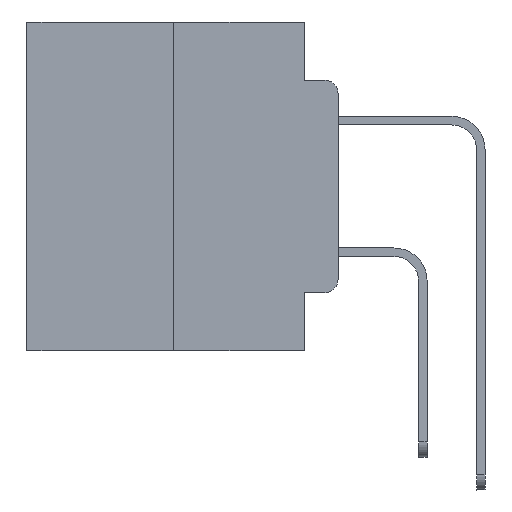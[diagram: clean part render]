
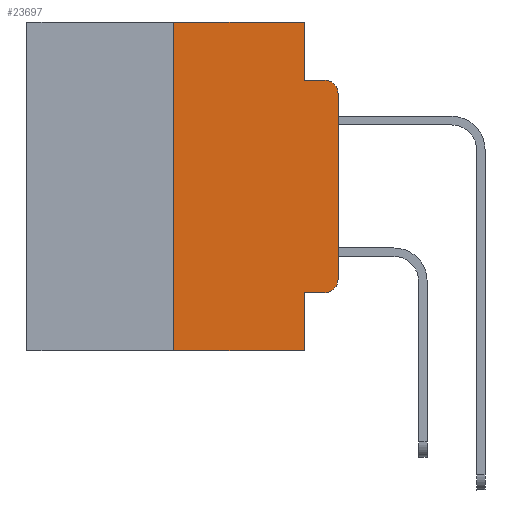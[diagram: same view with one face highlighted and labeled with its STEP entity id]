
A CAD part, left-side view. The second image highlights one B-rep face of the part: STEP entity #23697.
In plain terms, the highlighted planar face has unit normal (-1, 0, 0).
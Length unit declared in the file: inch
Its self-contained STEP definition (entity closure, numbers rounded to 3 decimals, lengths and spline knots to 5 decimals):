
#39 = CARTESIAN_POINT ( 'NONE',  ( 0., 0., -0.1085 ) ) ;
#104 = DIRECTION ( 'NONE',  ( 0., 0., -1. ) ) ;
#364 = VERTEX_POINT ( 'NONE', #5366 ) ;
#497 = CARTESIAN_POINT ( 'NONE',  ( 0., 0.473, -0.5 ) ) ;
#549 = VERTEX_POINT ( 'NONE', #11888 ) ;
#791 = DIRECTION ( 'NONE',  ( 0., 0., 1. ) ) ;
#1416 = CARTESIAN_POINT ( 'NONE',  ( 0., 0.02, -0.1085 ) ) ;
#1719 = VECTOR ( 'NONE', #791, 39.37008 ) ;
#1750 = EDGE_CURVE ( 'NONE', #549, #17195, #18834, .T. ) ;
#2584 = VECTOR ( 'NONE', #20790, 39.37008 ) ;
#2602 = LINE ( 'NONE', #497, #24653 ) ;
#3298 = ORIENTED_EDGE ( 'NONE', *, *, #20959, .F. ) ;
#3599 = DIRECTION ( 'NONE',  ( 0., 0., -1. ) ) ;
#3715 = CARTESIAN_POINT ( 'NONE',  ( 0., 0., -0.3915 ) ) ;
#3893 = CARTESIAN_POINT ( 'NONE',  ( 0., 0.051, -0.4115 ) ) ;
#4524 = VERTEX_POINT ( 'NONE', #39 ) ;
#4659 = EDGE_CURVE ( 'NONE', #364, #6423, #24624, .T. ) ;
#4721 = DIRECTION ( 'NONE',  ( 1., 0., 0. ) ) ;
#5366 = CARTESIAN_POINT ( 'NONE',  ( 0., 0.051, 0. ) ) ;
#5656 = ORIENTED_EDGE ( 'NONE', *, *, #24674, .T. ) ;
#5725 = LINE ( 'NONE', #25254, #16434 ) ;
#6086 = DIRECTION ( 'NONE',  ( 0., -1., 0. ) ) ;
#6367 = VERTEX_POINT ( 'NONE', #10604 ) ;
#6423 = VERTEX_POINT ( 'NONE', #6450 ) ;
#6450 = CARTESIAN_POINT ( 'NONE',  ( 0., 0.051, -0.0885 ) ) ;
#6804 = DIRECTION ( 'NONE',  ( 0., -1., 0. ) ) ;
#7242 = EDGE_CURVE ( 'NONE', #549, #13559, #2602, .T. ) ;
#7715 = ORIENTED_EDGE ( 'NONE', *, *, #1750, .F. ) ;
#8361 = EDGE_CURVE ( 'NONE', #17195, #364, #19679, .T. ) ;
#8904 = CARTESIAN_POINT ( 'NONE',  ( 0., 0.051, -0.0885 ) ) ;
#9070 = VERTEX_POINT ( 'NONE', #3715 ) ;
#9208 = VERTEX_POINT ( 'NONE', #27533 ) ;
#9898 = LINE ( 'NONE', #3893, #14875 ) ;
#10419 = ORIENTED_EDGE ( 'NONE', *, *, #13565, .T. ) ;
#10469 = EDGE_CURVE ( 'NONE', #6423, #10870, #12229, .T. ) ;
#10604 = CARTESIAN_POINT ( 'NONE',  ( 0., 0.051, -0.4115 ) ) ;
#10618 = CARTESIAN_POINT ( 'NONE',  ( 0., 0.02, -0.0885 ) ) ;
#10797 = EDGE_CURVE ( 'NONE', #6367, #9208, #9898, .T. ) ;
#10870 = VERTEX_POINT ( 'NONE', #10618 ) ;
#11125 = EDGE_LOOP ( 'NONE', ( #5656, #11391, #12055, #17701, #24044, #7715, #25335, #3298, #21060, #10419 ) ) ;
#11391 = ORIENTED_EDGE ( 'NONE', *, *, #20426, .T. ) ;
#11888 = CARTESIAN_POINT ( 'NONE',  ( 0., 0.25, -0.5 ) ) ;
#12055 = ORIENTED_EDGE ( 'NONE', *, *, #10469, .F. ) ;
#12229 = LINE ( 'NONE', #8904, #22877 ) ;
#12625 = VECTOR ( 'NONE', #13993, 39.37008 ) ;
#13042 = DIRECTION ( 'NONE',  ( -1., 0., 0. ) ) ;
#13264 = PLANE ( 'NONE',  #20012 ) ;
#13336 = VECTOR ( 'NONE', #17343, 39.37008 ) ;
#13559 = VERTEX_POINT ( 'NONE', #15093 ) ;
#13565 = EDGE_CURVE ( 'NONE', #9208, #9070, #22328, .T. ) ;
#13970 = CIRCLE ( 'NONE', #19260, 0.02 ) ;
#13993 = DIRECTION ( 'NONE',  ( 0., 0., -1. ) ) ;
#14875 = VECTOR ( 'NONE', #6086, 39.37008 ) ;
#15093 = CARTESIAN_POINT ( 'NONE',  ( 0., 0.051, -0.5 ) ) ;
#16434 = VECTOR ( 'NONE', #27340, 39.37008 ) ;
#16440 = DIRECTION ( 'NONE',  ( -1., 0., 0. ) ) ;
#17195 = VERTEX_POINT ( 'NONE', #22677 ) ;
#17343 = DIRECTION ( 'NONE',  ( 0., 0., -1. ) ) ;
#17437 = CARTESIAN_POINT ( 'NONE',  ( 0., 0.051, 0. ) ) ;
#17701 = ORIENTED_EDGE ( 'NONE', *, *, #4659, .F. ) ;
#18262 = LINE ( 'NONE', #26682, #12625 ) ;
#18643 = CARTESIAN_POINT ( 'NONE',  ( 0., 0.473, 0. ) ) ;
#18834 = LINE ( 'NONE', #22906, #1719 ) ;
#19188 = FACE_OUTER_BOUND ( 'NONE', #11125, .T. ) ;
#19260 = AXIS2_PLACEMENT_3D ( 'NONE', #1416, #16440, #3599 ) ;
#19679 = LINE ( 'NONE', #18643, #2584 ) ;
#19684 = DIRECTION ( 'NONE',  ( 0., 0., -1. ) ) ;
#19835 = DIRECTION ( 'NONE',  ( 0., -1., 0. ) ) ;
#20012 = AXIS2_PLACEMENT_3D ( 'NONE', #23872, #4721, #19684 ) ;
#20022 = AXIS2_PLACEMENT_3D ( 'NONE', #25741, #13042, #104 ) ;
#20426 = EDGE_CURVE ( 'NONE', #4524, #10870, #13970, .T. ) ;
#20790 = DIRECTION ( 'NONE',  ( 0., -1., 0. ) ) ;
#20959 = EDGE_CURVE ( 'NONE', #6367, #13559, #18262, .T. ) ;
#21060 = ORIENTED_EDGE ( 'NONE', *, *, #10797, .T. ) ;
#22328 = CIRCLE ( 'NONE', #20022, 0.02 ) ;
#22677 = CARTESIAN_POINT ( 'NONE',  ( 0., 0.25, 0. ) ) ;
#22877 = VECTOR ( 'NONE', #6804, 39.37008 ) ;
#22906 = CARTESIAN_POINT ( 'NONE',  ( 0., 0.25, 0. ) ) ;
#23697 = ADVANCED_FACE ( 'NONE', ( #19188 ), #13264, .F. ) ;
#23872 = CARTESIAN_POINT ( 'NONE',  ( 0., 0.473, 0. ) ) ;
#24044 = ORIENTED_EDGE ( 'NONE', *, *, #8361, .F. ) ;
#24624 = LINE ( 'NONE', #17437, #13336 ) ;
#24653 = VECTOR ( 'NONE', #19835, 39.37008 ) ;
#24674 = EDGE_CURVE ( 'NONE', #9070, #4524, #5725, .T. ) ;
#25254 = CARTESIAN_POINT ( 'NONE',  ( 0., 0., 0. ) ) ;
#25335 = ORIENTED_EDGE ( 'NONE', *, *, #7242, .T. ) ;
#25741 = CARTESIAN_POINT ( 'NONE',  ( 0., 0.02, -0.3915 ) ) ;
#26682 = CARTESIAN_POINT ( 'NONE',  ( 0., 0.051, 0. ) ) ;
#27340 = DIRECTION ( 'NONE',  ( 0., 0., 1. ) ) ;
#27533 = CARTESIAN_POINT ( 'NONE',  ( 0., 0.02, -0.4115 ) ) ;
